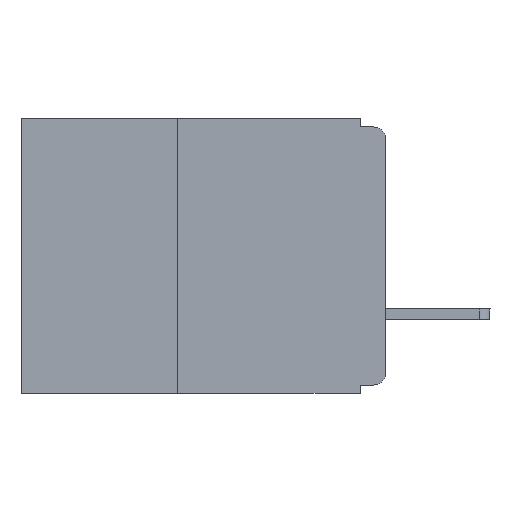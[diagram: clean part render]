
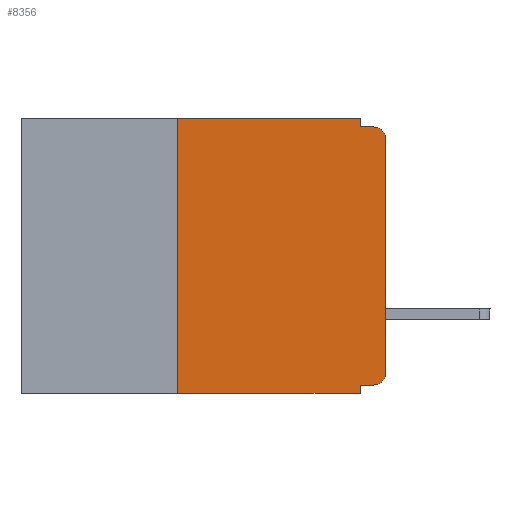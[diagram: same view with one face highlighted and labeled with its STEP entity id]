
A CAD part, left-side view. The second image highlights one B-rep face of the part: STEP entity #8356.
In plain terms, the highlighted planar face has unit normal (-1, 0, 0).
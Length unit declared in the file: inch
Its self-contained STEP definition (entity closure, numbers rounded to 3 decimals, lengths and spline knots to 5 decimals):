
#8 = DIRECTION ( 'NONE',  ( 1., 0., 0. ) ) ;
#66 = VERTEX_POINT ( 'NONE', #1797 ) ;
#293 = DIRECTION ( 'NONE',  ( 0., 0., -1. ) ) ;
#411 = CARTESIAN_POINT ( 'NONE',  ( 0., 0.25, 0. ) ) ;
#427 = LINE ( 'NONE', #3275, #9457 ) ;
#494 = CARTESIAN_POINT ( 'NONE',  ( 0., 0.031, -0.32 ) ) ;
#637 = ORIENTED_EDGE ( 'NONE', *, *, #3296, .F. ) ;
#718 = CARTESIAN_POINT ( 'NONE',  ( 0., 0., -0.32 ) ) ;
#727 = LINE ( 'NONE', #1564, #2163 ) ;
#864 = VECTOR ( 'NONE', #6804, 39.37008 ) ;
#875 = EDGE_CURVE ( 'NONE', #7119, #8206, #8918, .T. ) ;
#1069 = EDGE_CURVE ( 'NONE', #9702, #66, #1146, .T. ) ;
#1146 = LINE ( 'NONE', #2951, #9942 ) ;
#1319 = CARTESIAN_POINT ( 'NONE',  ( 0., 0.031, -0.33 ) ) ;
#1564 = CARTESIAN_POINT ( 'NONE',  ( 0., 0.437, 0. ) ) ;
#1660 = PLANE ( 'NONE',  #3108 ) ;
#1797 = CARTESIAN_POINT ( 'NONE',  ( 0., 0., -0.025 ) ) ;
#1815 = CARTESIAN_POINT ( 'NONE',  ( 0., 0., -0.305 ) ) ;
#1920 = CARTESIAN_POINT ( 'NONE',  ( 0., 0.031, 0. ) ) ;
#2057 = AXIS2_PLACEMENT_3D ( 'NONE', #2866, #8781, #4469 ) ;
#2113 = ORIENTED_EDGE ( 'NONE', *, *, #4487, .F. ) ;
#2163 = VECTOR ( 'NONE', #10676, 39.37008 ) ;
#2519 = ORIENTED_EDGE ( 'NONE', *, *, #7498, .F. ) ;
#2866 = CARTESIAN_POINT ( 'NONE',  ( 0., 0.015, -0.025 ) ) ;
#2951 = CARTESIAN_POINT ( 'NONE',  ( 0., 0., 0. ) ) ;
#3108 = AXIS2_PLACEMENT_3D ( 'NONE', #4113, #8, #9980 ) ;
#3129 = ORIENTED_EDGE ( 'NONE', *, *, #6076, .F. ) ;
#3275 = CARTESIAN_POINT ( 'NONE',  ( 0., 0.25, -0.33 ) ) ;
#3296 = EDGE_CURVE ( 'NONE', #6739, #9718, #5195, .T. ) ;
#3533 = ORIENTED_EDGE ( 'NONE', *, *, #10644, .F. ) ;
#3812 = DIRECTION ( 'NONE',  ( 0., 0., 1. ) ) ;
#3964 = ORIENTED_EDGE ( 'NONE', *, *, #8945, .T. ) ;
#4066 = CARTESIAN_POINT ( 'NONE',  ( 0., 0.015, -0.01 ) ) ;
#4094 = LINE ( 'NONE', #9444, #9604 ) ;
#4113 = CARTESIAN_POINT ( 'NONE',  ( 0., 0.437, 0. ) ) ;
#4329 = CARTESIAN_POINT ( 'NONE',  ( 0., 0.031, -0.01 ) ) ;
#4406 = FACE_OUTER_BOUND ( 'NONE', #10765, .T. ) ;
#4469 = DIRECTION ( 'NONE',  ( 0., 0., -1. ) ) ;
#4487 = EDGE_CURVE ( 'NONE', #7896, #8206, #7408, .T. ) ;
#4540 = EDGE_CURVE ( 'NONE', #6329, #6739, #727, .T. ) ;
#4674 = DIRECTION ( 'NONE',  ( 0., 0., -1. ) ) ;
#4868 = AXIS2_PLACEMENT_3D ( 'NONE', #6922, #10255, #293 ) ;
#5087 = CARTESIAN_POINT ( 'NONE',  ( 0., 0.031, 0. ) ) ;
#5115 = ORIENTED_EDGE ( 'NONE', *, *, #6926, .T. ) ;
#5195 = LINE ( 'NONE', #5087, #864 ) ;
#5524 = ORIENTED_EDGE ( 'NONE', *, *, #4540, .F. ) ;
#5557 = VECTOR ( 'NONE', #6520, 39.37008 ) ;
#5667 = VERTEX_POINT ( 'NONE', #4066 ) ;
#5810 = CARTESIAN_POINT ( 'NONE',  ( 0., 0.015, -0.32 ) ) ;
#6036 = DIRECTION ( 'NONE',  ( 0., -1., 0. ) ) ;
#6076 = EDGE_CURVE ( 'NONE', #7119, #6329, #427, .T. ) ;
#6329 = VERTEX_POINT ( 'NONE', #411 ) ;
#6393 = CIRCLE ( 'NONE', #4868, 0.015 ) ;
#6520 = DIRECTION ( 'NONE',  ( 0., 1., 0. ) ) ;
#6666 = VERTEX_POINT ( 'NONE', #5810 ) ;
#6698 = VECTOR ( 'NONE', #6036, 39.37008 ) ;
#6739 = VERTEX_POINT ( 'NONE', #1920 ) ;
#6804 = DIRECTION ( 'NONE',  ( 0., 0., -1. ) ) ;
#6922 = CARTESIAN_POINT ( 'NONE',  ( 0., 0.015, -0.305 ) ) ;
#6926 = EDGE_CURVE ( 'NONE', #66, #5667, #9055, .T. ) ;
#7119 = VERTEX_POINT ( 'NONE', #9010 ) ;
#7408 = LINE ( 'NONE', #1319, #9240 ) ;
#7498 = EDGE_CURVE ( 'NONE', #6666, #7896, #8979, .T. ) ;
#7853 = ORIENTED_EDGE ( 'NONE', *, *, #1069, .T. ) ;
#7896 = VERTEX_POINT ( 'NONE', #494 ) ;
#8206 = VERTEX_POINT ( 'NONE', #8294 ) ;
#8294 = CARTESIAN_POINT ( 'NONE',  ( 0., 0.031, -0.33 ) ) ;
#8356 = ADVANCED_FACE ( 'NONE', ( #4406 ), #1660, .F. ) ;
#8578 = DIRECTION ( 'NONE',  ( 0., -1., 0. ) ) ;
#8781 = DIRECTION ( 'NONE',  ( -1., 0., 0. ) ) ;
#8918 = LINE ( 'NONE', #10058, #6698 ) ;
#8945 = EDGE_CURVE ( 'NONE', #6666, #9702, #6393, .T. ) ;
#8979 = LINE ( 'NONE', #718, #5557 ) ;
#9010 = CARTESIAN_POINT ( 'NONE',  ( 0., 0.25, -0.33 ) ) ;
#9055 = CIRCLE ( 'NONE', #2057, 0.015 ) ;
#9156 = DIRECTION ( 'NONE',  ( 0., 0., 1. ) ) ;
#9240 = VECTOR ( 'NONE', #4674, 39.37008 ) ;
#9444 = CARTESIAN_POINT ( 'NONE',  ( 0., 0., -0.01 ) ) ;
#9457 = VECTOR ( 'NONE', #9156, 39.37008 ) ;
#9604 = VECTOR ( 'NONE', #8578, 39.37008 ) ;
#9616 = ORIENTED_EDGE ( 'NONE', *, *, #875, .T. ) ;
#9702 = VERTEX_POINT ( 'NONE', #1815 ) ;
#9718 = VERTEX_POINT ( 'NONE', #4329 ) ;
#9942 = VECTOR ( 'NONE', #3812, 39.37008 ) ;
#9980 = DIRECTION ( 'NONE',  ( 0., 0., -1. ) ) ;
#10058 = CARTESIAN_POINT ( 'NONE',  ( 0., 0.437, -0.33 ) ) ;
#10255 = DIRECTION ( 'NONE',  ( -1., 0., 0. ) ) ;
#10644 = EDGE_CURVE ( 'NONE', #9718, #5667, #4094, .T. ) ;
#10676 = DIRECTION ( 'NONE',  ( 0., -1., 0. ) ) ;
#10765 = EDGE_LOOP ( 'NONE', ( #7853, #5115, #3533, #637, #5524, #3129, #9616, #2113, #2519, #3964 ) ) ;
